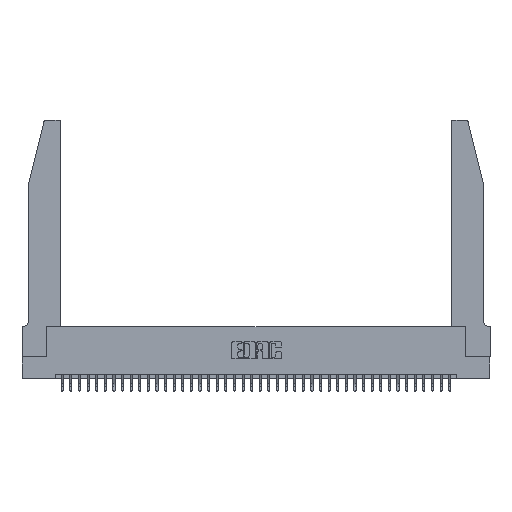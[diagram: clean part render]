
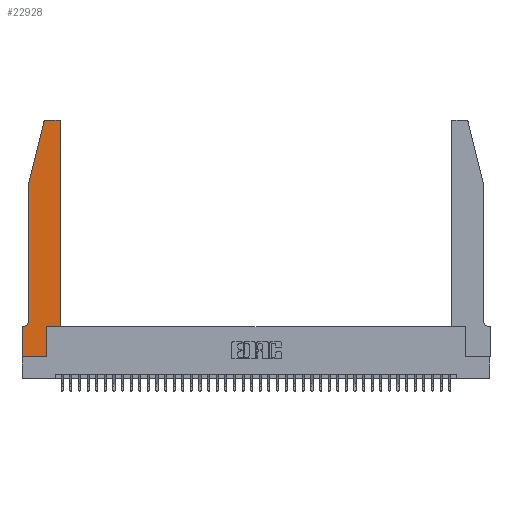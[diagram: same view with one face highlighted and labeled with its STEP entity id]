
A CAD part, top view. The second image highlights one B-rep face of the part: STEP entity #22928.
In plain terms, the highlighted planar face has unit normal (0, 0, 1).
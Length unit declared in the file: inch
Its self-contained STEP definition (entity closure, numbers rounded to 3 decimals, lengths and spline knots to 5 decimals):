
#1045 = DIRECTION ( 'NONE',  ( 0., 0., 1. ) ) ;
#1073 = VERTEX_POINT ( 'NONE', #12839 ) ;
#1634 = AXIS2_PLACEMENT_3D ( 'NONE', #19959, #1045, #23095 ) ;
#1772 = VERTEX_POINT ( 'NONE', #9619 ) ;
#2913 = DIRECTION ( 'NONE',  ( 1., 0., 0. ) ) ;
#3720 = CIRCLE ( 'NONE', #24838, 0.07 ) ;
#4784 = ORIENTED_EDGE ( 'NONE', *, *, #29972, .T. ) ;
#5128 = CARTESIAN_POINT ( 'NONE',  ( 0., 0., 0.37 ) ) ;
#5259 = ORIENTED_EDGE ( 'NONE', *, *, #35276, .T. ) ;
#6342 = DIRECTION ( 'NONE',  ( 0., -1., 0. ) ) ;
#8633 = DIRECTION ( 'NONE',  ( 0., 0., -1. ) ) ;
#8667 = CARTESIAN_POINT ( 'NONE',  ( 0.4205, 2.72, 0.37 ) ) ;
#9008 = DIRECTION ( 'NONE',  ( 0., -1., 0. ) ) ;
#9303 = CARTESIAN_POINT ( 'NONE',  ( 0.0755, 0.35, 0.37 ) ) ;
#9619 = CARTESIAN_POINT ( 'NONE',  ( 0.4505, 2.72, 0.37 ) ) ;
#10265 = ORIENTED_EDGE ( 'NONE', *, *, #21428, .T. ) ;
#10741 = ORIENTED_EDGE ( 'NONE', *, *, #30901, .T. ) ;
#11014 = CARTESIAN_POINT ( 'NONE',  ( 0.2865, 0., 0.37 ) ) ;
#11303 = LINE ( 'NONE', #38987, #19629 ) ;
#11425 = VERTEX_POINT ( 'NONE', #26585 ) ;
#11843 = DIRECTION ( 'NONE',  ( 1., 0., 0. ) ) ;
#12127 = VECTOR ( 'NONE', #19853, 39.37008 ) ;
#12149 = AXIS2_PLACEMENT_3D ( 'NONE', #40361, #21791, #2913 ) ;
#12839 = CARTESIAN_POINT ( 'NONE',  ( 0.0755, 0.42, 0.37 ) ) ;
#13304 = EDGE_CURVE ( 'NONE', #26293, #11425, #22476, .T. ) ;
#13565 = CARTESIAN_POINT ( 'NONE',  ( 0.2865, 0.35, 0.37 ) ) ;
#14118 = DIRECTION ( 'NONE',  ( 1., 0., 0. ) ) ;
#14786 = VECTOR ( 'NONE', #9008, 39.37008 ) ;
#14812 = LINE ( 'NONE', #33219, #37656 ) ;
#14878 = EDGE_LOOP ( 'NONE', ( #38985, #4784, #28818, #10265, #17608, #23930, #39455, #5259, #29300, #21003, #27323, #10741 ) ) ;
#15134 = LINE ( 'NONE', #30294, #30721 ) ;
#15523 = CARTESIAN_POINT ( 'NONE',  ( 0.0755, 2., 0.37 ) ) ;
#16142 = VECTOR ( 'NONE', #6342, 39.37008 ) ;
#17608 = ORIENTED_EDGE ( 'NONE', *, *, #34874, .T. ) ;
#17894 = DIRECTION ( 'NONE',  ( -0.239, -0.971, 0. ) ) ;
#17996 = CARTESIAN_POINT ( 'NONE',  ( 0.284, 2.75, 0.37 ) ) ;
#18573 = EDGE_CURVE ( 'NONE', #11425, #35481, #31360, .T. ) ;
#19597 = VERTEX_POINT ( 'NONE', #20456 ) ;
#19629 = VECTOR ( 'NONE', #14118, 39.37008 ) ;
#19853 = DIRECTION ( 'NONE',  ( 0., 1., 0. ) ) ;
#19959 = CARTESIAN_POINT ( 'NONE',  ( 0., 0.35, 0.37 ) ) ;
#20456 = CARTESIAN_POINT ( 'NONE',  ( 0.4205, 2.75, 0.37 ) ) ;
#21003 = ORIENTED_EDGE ( 'NONE', *, *, #33575, .T. ) ;
#21090 = CIRCLE ( 'NONE', #33587, 0.03 ) ;
#21428 = EDGE_CURVE ( 'NONE', #31021, #1073, #23456, .T. ) ;
#21720 = CARTESIAN_POINT ( 'NONE',  ( 0.4505, 0.35, 0.37 ) ) ;
#21791 = DIRECTION ( 'NONE',  ( 0., 0., 1. ) ) ;
#22476 = LINE ( 'NONE', #9303, #29788 ) ;
#22928 = ADVANCED_FACE ( 'NONE', ( #34012 ), #32346, .T. ) ;
#22941 = VERTEX_POINT ( 'NONE', #38551 ) ;
#22981 = LINE ( 'NONE', #23097, #30289 ) ;
#23095 = DIRECTION ( 'NONE',  ( 1., 0., 0. ) ) ;
#23097 = CARTESIAN_POINT ( 'NONE',  ( 0.4505, 0.35, 0.37 ) ) ;
#23456 = LINE ( 'NONE', #25101, #16142 ) ;
#23930 = ORIENTED_EDGE ( 'NONE', *, *, #13304, .T. ) ;
#23938 = DIRECTION ( 'NONE',  ( 1., 0., 0. ) ) ;
#24732 = CARTESIAN_POINT ( 'NONE',  ( 0., 0., 0.37 ) ) ;
#24838 = AXIS2_PLACEMENT_3D ( 'NONE', #27369, #8633, #30504 ) ;
#25101 = CARTESIAN_POINT ( 'NONE',  ( 0.0755, 2., 0.37 ) ) ;
#25606 = CARTESIAN_POINT ( 'NONE',  ( 0.2865, 0.35, 0.37 ) ) ;
#25767 = VERTEX_POINT ( 'NONE', #17996 ) ;
#26293 = VERTEX_POINT ( 'NONE', #33071 ) ;
#26333 = EDGE_CURVE ( 'NONE', #19597, #25767, #14812, .T. ) ;
#26585 = CARTESIAN_POINT ( 'NONE',  ( 0., 0.35, 0.37 ) ) ;
#26844 = EDGE_CURVE ( 'NONE', #27817, #30139, #36925, .T. ) ;
#27275 = VERTEX_POINT ( 'NONE', #21720 ) ;
#27323 = ORIENTED_EDGE ( 'NONE', *, *, #34115, .T. ) ;
#27369 = CARTESIAN_POINT ( 'NONE',  ( 0.0055, 0.42, 0.37 ) ) ;
#27817 = VERTEX_POINT ( 'NONE', #11014 ) ;
#28818 = ORIENTED_EDGE ( 'NONE', *, *, #34347, .T. ) ;
#29300 = ORIENTED_EDGE ( 'NONE', *, *, #26844, .T. ) ;
#29788 = VECTOR ( 'NONE', #37347, 39.37008 ) ;
#29972 = EDGE_CURVE ( 'NONE', #25767, #22941, #38655, .T. ) ;
#30139 = VERTEX_POINT ( 'NONE', #25606 ) ;
#30223 = DIRECTION ( 'NONE',  ( -1., 0., 0. ) ) ;
#30289 = VECTOR ( 'NONE', #32348, 39.37008 ) ;
#30294 = CARTESIAN_POINT ( 'NONE',  ( 0.0755, 2., 0.37 ) ) ;
#30504 = DIRECTION ( 'NONE',  ( -1., 0., 0. ) ) ;
#30536 = DIRECTION ( 'NONE',  ( 0., 0., 1. ) ) ;
#30651 = VECTOR ( 'NONE', #23938, 39.37008 ) ;
#30721 = VECTOR ( 'NONE', #17894, 39.37008 ) ;
#30901 = EDGE_CURVE ( 'NONE', #1772, #19597, #21090, .T. ) ;
#31021 = VERTEX_POINT ( 'NONE', #15523 ) ;
#31360 = LINE ( 'NONE', #36916, #14786 ) ;
#32346 = PLANE ( 'NONE',  #1634 ) ;
#32348 = DIRECTION ( 'NONE',  ( 0., 1., 0. ) ) ;
#33071 = CARTESIAN_POINT ( 'NONE',  ( 0.0055, 0.35, 0.37 ) ) ;
#33219 = CARTESIAN_POINT ( 'NONE',  ( 0.2605, 2.75, 0.37 ) ) ;
#33575 = EDGE_CURVE ( 'NONE', #30139, #27275, #11303, .T. ) ;
#33587 = AXIS2_PLACEMENT_3D ( 'NONE', #8667, #30536, #11843 ) ;
#34012 = FACE_OUTER_BOUND ( 'NONE', #14878, .T. ) ;
#34115 = EDGE_CURVE ( 'NONE', #27275, #1772, #22981, .T. ) ;
#34347 = EDGE_CURVE ( 'NONE', #22941, #31021, #15134, .T. ) ;
#34874 = EDGE_CURVE ( 'NONE', #1073, #26293, #3720, .T. ) ;
#35276 = EDGE_CURVE ( 'NONE', #35481, #27817, #39852, .T. ) ;
#35481 = VERTEX_POINT ( 'NONE', #24732 ) ;
#36916 = CARTESIAN_POINT ( 'NONE',  ( 0., 0., 0.37 ) ) ;
#36925 = LINE ( 'NONE', #13565, #12127 ) ;
#37347 = DIRECTION ( 'NONE',  ( -1., 0., 0. ) ) ;
#37656 = VECTOR ( 'NONE', #30223, 39.37008 ) ;
#38551 = CARTESIAN_POINT ( 'NONE',  ( 0.25487, 2.72718, 0.37 ) ) ;
#38655 = CIRCLE ( 'NONE', #12149, 0.03 ) ;
#38985 = ORIENTED_EDGE ( 'NONE', *, *, #26333, .T. ) ;
#38987 = CARTESIAN_POINT ( 'NONE',  ( 0.4505, 0.35, 0.37 ) ) ;
#39455 = ORIENTED_EDGE ( 'NONE', *, *, #18573, .T. ) ;
#39852 = LINE ( 'NONE', #5128, #30651 ) ;
#40361 = CARTESIAN_POINT ( 'NONE',  ( 0.284, 2.72, 0.37 ) ) ;
